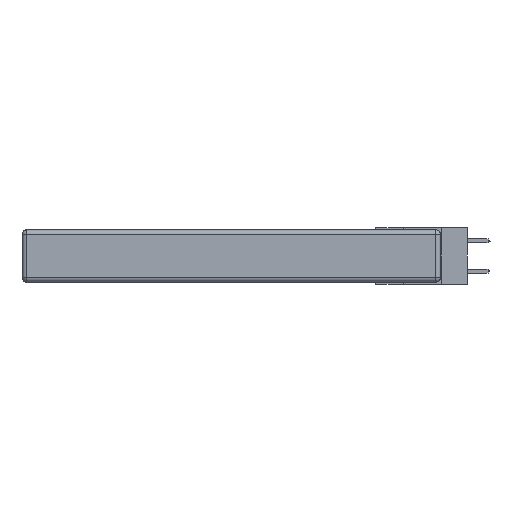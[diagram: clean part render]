
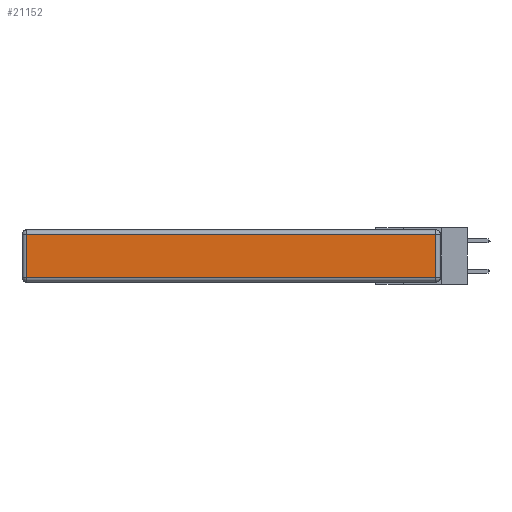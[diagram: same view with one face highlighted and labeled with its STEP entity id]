
A CAD part, left-side view. The second image highlights one B-rep face of the part: STEP entity #21152.
In plain terms, the highlighted planar face has unit normal (-1, 0, 0).
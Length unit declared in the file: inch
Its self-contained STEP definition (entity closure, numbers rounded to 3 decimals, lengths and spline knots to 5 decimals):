
#687 = ORIENTED_EDGE ( 'NONE', *, *, #28342, .T. ) ;
#1104 = CARTESIAN_POINT ( 'NONE',  ( 0., 2.72, -0.03 ) ) ;
#1815 = CARTESIAN_POINT ( 'NONE',  ( 0., 0.03, -0.313 ) ) ;
#2072 = DIRECTION ( 'NONE',  ( 0., 0., 1. ) ) ;
#3498 = DIRECTION ( 'NONE',  ( 0., 0., 1. ) ) ;
#4580 = ORIENTED_EDGE ( 'NONE', *, *, #25079, .T. ) ;
#5895 = LINE ( 'NONE', #13744, #29301 ) ;
#7309 = LINE ( 'NONE', #30427, #12431 ) ;
#7642 = CARTESIAN_POINT ( 'NONE',  ( 0., 0.03, -0.03 ) ) ;
#8341 = EDGE_LOOP ( 'NONE', ( #687, #21049, #4580, #27163 ) ) ;
#8781 = AXIS2_PLACEMENT_3D ( 'NONE', #27036, #31928, #2072 ) ;
#8785 = DIRECTION ( 'NONE',  ( 0., 1., 0. ) ) ;
#8912 = EDGE_CURVE ( 'NONE', #22686, #29438, #23890, .T. ) ;
#9477 = FACE_OUTER_BOUND ( 'NONE', #8341, .T. ) ;
#12431 = VECTOR ( 'NONE', #3498, 39.37008 ) ;
#13744 = CARTESIAN_POINT ( 'NONE',  ( 0., 2.75, -0.03 ) ) ;
#16062 = VERTEX_POINT ( 'NONE', #7642 ) ;
#19938 = VERTEX_POINT ( 'NONE', #1815 ) ;
#20220 = CARTESIAN_POINT ( 'NONE',  ( 0., 2.72, -0.343 ) ) ;
#21049 = ORIENTED_EDGE ( 'NONE', *, *, #31024, .T. ) ;
#21152 = ADVANCED_FACE ( 'NONE', ( #9477 ), #24349, .T. ) ;
#21236 = CARTESIAN_POINT ( 'NONE',  ( 0., 0., -0.313 ) ) ;
#22686 = VERTEX_POINT ( 'NONE', #1104 ) ;
#22693 = LINE ( 'NONE', #21236, #29302 ) ;
#23890 = LINE ( 'NONE', #20220, #28925 ) ;
#23950 = CARTESIAN_POINT ( 'NONE',  ( 0., 2.72, -0.313 ) ) ;
#24349 = PLANE ( 'NONE',  #8781 ) ;
#25079 = EDGE_CURVE ( 'NONE', #16062, #22686, #5895, .T. ) ;
#27036 = CARTESIAN_POINT ( 'NONE',  ( 0., 0., -0.343 ) ) ;
#27163 = ORIENTED_EDGE ( 'NONE', *, *, #8912, .T. ) ;
#27886 = DIRECTION ( 'NONE',  ( 0., 0., -1. ) ) ;
#28342 = EDGE_CURVE ( 'NONE', #29438, #19938, #22693, .T. ) ;
#28925 = VECTOR ( 'NONE', #27886, 39.37008 ) ;
#29301 = VECTOR ( 'NONE', #8785, 39.37008 ) ;
#29302 = VECTOR ( 'NONE', #30993, 39.37008 ) ;
#29438 = VERTEX_POINT ( 'NONE', #23950 ) ;
#30427 = CARTESIAN_POINT ( 'NONE',  ( 0., 0.03, -0.343 ) ) ;
#30993 = DIRECTION ( 'NONE',  ( 0., -1., 0. ) ) ;
#31024 = EDGE_CURVE ( 'NONE', #19938, #16062, #7309, .T. ) ;
#31928 = DIRECTION ( 'NONE',  ( -1., 0., 0. ) ) ;
